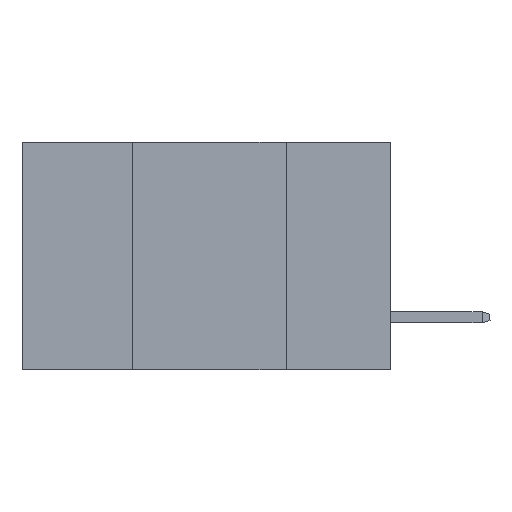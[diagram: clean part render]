
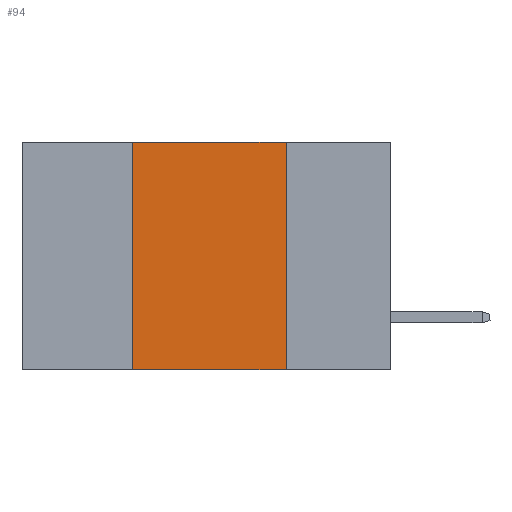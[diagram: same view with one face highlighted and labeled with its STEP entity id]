
A CAD part, left-side view. The second image highlights one B-rep face of the part: STEP entity #94.
In plain terms, the highlighted planar face has unit normal (-1, 0, 0).
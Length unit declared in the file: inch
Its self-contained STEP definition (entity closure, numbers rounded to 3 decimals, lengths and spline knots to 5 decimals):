
#94 = ADVANCED_FACE ( 'NONE', ( #14091 ), #7828, .F. ) ;
#532 = CARTESIAN_POINT ( 'NONE',  ( 0., 0.42, 0. ) ) ;
#1258 = CARTESIAN_POINT ( 'NONE',  ( 0., 0.17, 0. ) ) ;
#1416 = VECTOR ( 'NONE', #6994, 39.37008 ) ;
#1459 = ORIENTED_EDGE ( 'NONE', *, *, #17893, .F. ) ;
#3171 = LINE ( 'NONE', #3305, #19057 ) ;
#3274 = CARTESIAN_POINT ( 'NONE',  ( 0., 0.6, 0. ) ) ;
#3305 = CARTESIAN_POINT ( 'NONE',  ( 0., 0.6, 0. ) ) ;
#4477 = VECTOR ( 'NONE', #13090, 39.37008 ) ;
#5046 = CARTESIAN_POINT ( 'NONE',  ( 0., 0.42, 0. ) ) ;
#5779 = VERTEX_POINT ( 'NONE', #6757 ) ;
#6757 = CARTESIAN_POINT ( 'NONE',  ( 0., 0.17, -0.37 ) ) ;
#6994 = DIRECTION ( 'NONE',  ( 0., -1., 0. ) ) ;
#7004 = LINE ( 'NONE', #532, #15184 ) ;
#7828 = PLANE ( 'NONE',  #8338 ) ;
#8338 = AXIS2_PLACEMENT_3D ( 'NONE', #3274, #19108, #19902 ) ;
#8696 = EDGE_CURVE ( 'NONE', #10983, #5779, #21217, .T. ) ;
#10267 = EDGE_LOOP ( 'NONE', ( #19617, #15428, #1459, #19744 ) ) ;
#10983 = VERTEX_POINT ( 'NONE', #12723 ) ;
#11001 = CARTESIAN_POINT ( 'NONE',  ( 0., 0.42, -0.37 ) ) ;
#11949 = EDGE_CURVE ( 'NONE', #15831, #5779, #18433, .T. ) ;
#12723 = CARTESIAN_POINT ( 'NONE',  ( 0., 0.17, 0. ) ) ;
#13090 = DIRECTION ( 'NONE',  ( 0., 0., -1. ) ) ;
#14059 = DIRECTION ( 'NONE',  ( 0., 0., 1. ) ) ;
#14091 = FACE_OUTER_BOUND ( 'NONE', #10267, .T. ) ;
#14185 = EDGE_CURVE ( 'NONE', #19800, #10983, #3171, .T. ) ;
#15184 = VECTOR ( 'NONE', #14059, 39.37008 ) ;
#15428 = ORIENTED_EDGE ( 'NONE', *, *, #14185, .F. ) ;
#15831 = VERTEX_POINT ( 'NONE', #11001 ) ;
#17893 = EDGE_CURVE ( 'NONE', #15831, #19800, #7004, .T. ) ;
#18433 = LINE ( 'NONE', #19799, #1416 ) ;
#19057 = VECTOR ( 'NONE', #21184, 39.37008 ) ;
#19108 = DIRECTION ( 'NONE',  ( 1., 0., 0. ) ) ;
#19617 = ORIENTED_EDGE ( 'NONE', *, *, #8696, .F. ) ;
#19744 = ORIENTED_EDGE ( 'NONE', *, *, #11949, .T. ) ;
#19799 = CARTESIAN_POINT ( 'NONE',  ( 0., 0.6, -0.37 ) ) ;
#19800 = VERTEX_POINT ( 'NONE', #5046 ) ;
#19902 = DIRECTION ( 'NONE',  ( 0., 0., -1. ) ) ;
#21184 = DIRECTION ( 'NONE',  ( 0., -1., 0. ) ) ;
#21217 = LINE ( 'NONE', #1258, #4477 ) ;
